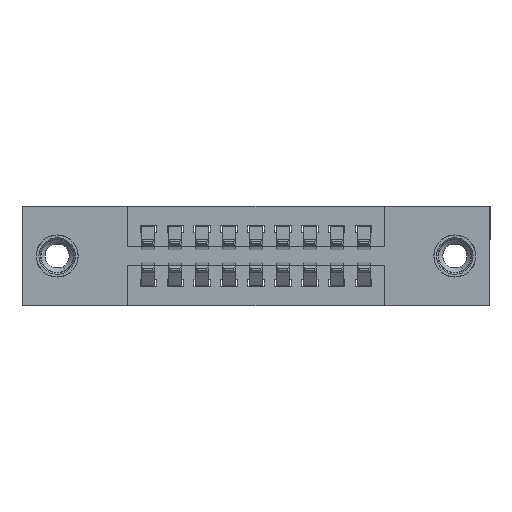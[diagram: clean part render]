
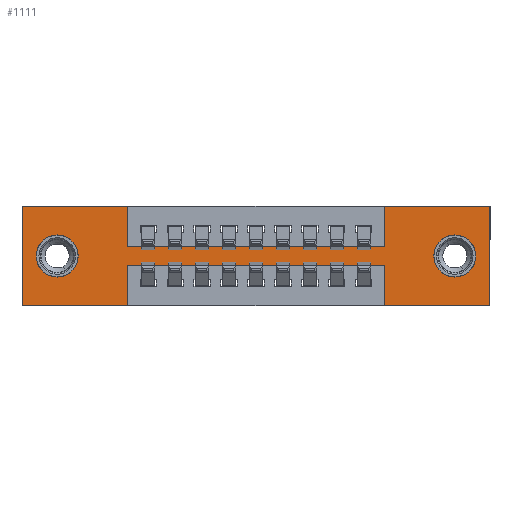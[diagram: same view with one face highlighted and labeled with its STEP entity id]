
A CAD part, front view. The second image highlights one B-rep face of the part: STEP entity #1111.
In plain terms, the highlighted planar face has unit normal (0, -1, 0).
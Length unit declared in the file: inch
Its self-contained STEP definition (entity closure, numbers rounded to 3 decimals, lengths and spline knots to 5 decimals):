
#207 = CARTESIAN_POINT ( 'NONE',  ( 1.3425, 0., -0.37 ) ) ;
#252 = DIRECTION ( 'NONE',  ( 1., 0., 0. ) ) ;
#415 = EDGE_CURVE ( 'NONE', #15424, #10336, #16353, .T. ) ;
#437 = CARTESIAN_POINT ( 'NONE',  ( 1.735, 0., 0. ) ) ;
#595 = ORIENTED_EDGE ( 'NONE', *, *, #5050, .F. ) ;
#692 = CARTESIAN_POINT ( 'NONE',  ( 1.605, 0., -0.263 ) ) ;
#884 = ORIENTED_EDGE ( 'NONE', *, *, #9360, .F. ) ;
#893 = CARTESIAN_POINT ( 'NONE',  ( 1.605, 0., -0.107 ) ) ;
#1111 = ADVANCED_FACE ( 'NONE', ( #7993, #14321, #15718 ), #10980, .T. ) ;
#1293 = AXIS2_PLACEMENT_3D ( 'NONE', #15008, #7419, #13548 ) ;
#1509 = CIRCLE ( 'NONE', #12187, 0.078 ) ;
#1554 = LINE ( 'NONE', #8705, #8069 ) ;
#1849 = CARTESIAN_POINT ( 'NONE',  ( 0., 0., -0.37 ) ) ;
#1929 = CIRCLE ( 'NONE', #10089, 0.078 ) ;
#1953 = VERTEX_POINT ( 'NONE', #10469 ) ;
#1966 = DIRECTION ( 'NONE',  ( -1., 0., 0. ) ) ;
#1985 = DIRECTION ( 'NONE',  ( 0., 0., -1. ) ) ;
#2085 = VECTOR ( 'NONE', #12582, 39.37008 ) ;
#2090 = CARTESIAN_POINT ( 'NONE',  ( 0., 0., -0.37 ) ) ;
#2304 = DIRECTION ( 'NONE',  ( 0., 0., 1. ) ) ;
#2460 = ORIENTED_EDGE ( 'NONE', *, *, #13533, .F. ) ;
#2558 = VECTOR ( 'NONE', #2304, 39.37008 ) ;
#2909 = CARTESIAN_POINT ( 'NONE',  ( 0.3925, 0., -0.22 ) ) ;
#2970 = EDGE_CURVE ( 'NONE', #9337, #15167, #8326, .T. ) ;
#2982 = VERTEX_POINT ( 'NONE', #7199 ) ;
#3263 = DIRECTION ( 'NONE',  ( 0., 0., -1. ) ) ;
#3488 = CARTESIAN_POINT ( 'NONE',  ( 1.605, 0., -0.185 ) ) ;
#3556 = LINE ( 'NONE', #6065, #2558 ) ;
#3629 = DIRECTION ( 'NONE',  ( 0., 0., 1. ) ) ;
#3724 = EDGE_CURVE ( 'NONE', #8773, #15424, #9285, .T. ) ;
#3735 = EDGE_LOOP ( 'NONE', ( #5140, #8130 ) ) ;
#3769 = LINE ( 'NONE', #6509, #15847 ) ;
#3925 = CARTESIAN_POINT ( 'NONE',  ( 1.605, 0., -0.185 ) ) ;
#4067 = EDGE_CURVE ( 'NONE', #6434, #2982, #3769, .T. ) ;
#4069 = DIRECTION ( 'NONE',  ( 0., 1., 0. ) ) ;
#4116 = ORIENTED_EDGE ( 'NONE', *, *, #13829, .F. ) ;
#4537 = VECTOR ( 'NONE', #3263, 39.37008 ) ;
#4695 = LINE ( 'NONE', #15962, #12978 ) ;
#4753 = EDGE_CURVE ( 'NONE', #15594, #6434, #3556, .T. ) ;
#4817 = VECTOR ( 'NONE', #13464, 39.37008 ) ;
#4844 = VECTOR ( 'NONE', #252, 39.37008 ) ;
#4912 = CIRCLE ( 'NONE', #10466, 0.078 ) ;
#5050 = EDGE_CURVE ( 'NONE', #7276, #15594, #13015, .T. ) ;
#5140 = ORIENTED_EDGE ( 'NONE', *, *, #2970, .T. ) ;
#5389 = ORIENTED_EDGE ( 'NONE', *, *, #10647, .F. ) ;
#5525 = CARTESIAN_POINT ( 'NONE',  ( 1.735, 0., -0.37 ) ) ;
#5573 = DIRECTION ( 'NONE',  ( -1., 0., 0. ) ) ;
#5698 = ORIENTED_EDGE ( 'NONE', *, *, #3724, .F. ) ;
#5729 = EDGE_CURVE ( 'NONE', #14629, #13542, #1929, .T. ) ;
#5925 = DIRECTION ( 'NONE',  ( 0., 1., 0. ) ) ;
#6063 = CARTESIAN_POINT ( 'NONE',  ( 0.13, 0., -0.263 ) ) ;
#6065 = CARTESIAN_POINT ( 'NONE',  ( 0., 0., 0. ) ) ;
#6308 = DIRECTION ( 'NONE',  ( 0., 0., -1. ) ) ;
#6364 = ORIENTED_EDGE ( 'NONE', *, *, #415, .F. ) ;
#6434 = VERTEX_POINT ( 'NONE', #12138 ) ;
#6509 = CARTESIAN_POINT ( 'NONE',  ( 0., 0., 0. ) ) ;
#7124 = ORIENTED_EDGE ( 'NONE', *, *, #16138, .F. ) ;
#7172 = CARTESIAN_POINT ( 'NONE',  ( 0.13, 0., -0.185 ) ) ;
#7199 = CARTESIAN_POINT ( 'NONE',  ( 0.3925, 0., 0. ) ) ;
#7224 = CARTESIAN_POINT ( 'NONE',  ( 0.13, 0., -0.107 ) ) ;
#7228 = VECTOR ( 'NONE', #11682, 39.37008 ) ;
#7276 = VERTEX_POINT ( 'NONE', #14597 ) ;
#7419 = DIRECTION ( 'NONE',  ( 0., -1., 0. ) ) ;
#7774 = VERTEX_POINT ( 'NONE', #8724 ) ;
#7982 = ORIENTED_EDGE ( 'NONE', *, *, #4067, .F. ) ;
#7993 = FACE_BOUND ( 'NONE', #3735, .T. ) ;
#8042 = EDGE_LOOP ( 'NONE', ( #13477, #9105 ) ) ;
#8069 = VECTOR ( 'NONE', #3629, 39.37008 ) ;
#8118 = CARTESIAN_POINT ( 'NONE',  ( 0.3925, 0., -0.15 ) ) ;
#8130 = ORIENTED_EDGE ( 'NONE', *, *, #15494, .T. ) ;
#8326 = CIRCLE ( 'NONE', #8721, 0.078 ) ;
#8705 = CARTESIAN_POINT ( 'NONE',  ( 1.3425, 0., 0. ) ) ;
#8721 = AXIS2_PLACEMENT_3D ( 'NONE', #3488, #5925, #1985 ) ;
#8724 = CARTESIAN_POINT ( 'NONE',  ( 1.3425, 0., -0.15 ) ) ;
#8773 = VERTEX_POINT ( 'NONE', #5525 ) ;
#8974 = DIRECTION ( 'NONE',  ( 1., 0., 0. ) ) ;
#9105 = ORIENTED_EDGE ( 'NONE', *, *, #13437, .T. ) ;
#9285 = LINE ( 'NONE', #1849, #12857 ) ;
#9337 = VERTEX_POINT ( 'NONE', #893 ) ;
#9360 = EDGE_CURVE ( 'NONE', #1953, #7774, #16151, .T. ) ;
#9553 = ORIENTED_EDGE ( 'NONE', *, *, #12789, .F. ) ;
#9577 = DIRECTION ( 'NONE',  ( 0., 0., 1. ) ) ;
#9854 = VECTOR ( 'NONE', #1966, 39.37008 ) ;
#9967 = LINE ( 'NONE', #437, #7228 ) ;
#10028 = VECTOR ( 'NONE', #5573, 39.37008 ) ;
#10089 = AXIS2_PLACEMENT_3D ( 'NONE', #15545, #4069, #12922 ) ;
#10190 = CARTESIAN_POINT ( 'NONE',  ( 1.3425, 0., -0.37 ) ) ;
#10324 = ORIENTED_EDGE ( 'NONE', *, *, #4753, .F. ) ;
#10336 = VERTEX_POINT ( 'NONE', #10549 ) ;
#10445 = VERTEX_POINT ( 'NONE', #11400 ) ;
#10466 = AXIS2_PLACEMENT_3D ( 'NONE', #7172, #16143, #9577 ) ;
#10469 = CARTESIAN_POINT ( 'NONE',  ( 0.3925, 0., -0.15 ) ) ;
#10481 = EDGE_LOOP ( 'NONE', ( #9553, #4116, #6364, #5698, #7124, #5389, #2460, #884, #12987, #7982, #10324, #595 ) ) ;
#10549 = CARTESIAN_POINT ( 'NONE',  ( 1.3425, 0., -0.22 ) ) ;
#10647 = EDGE_CURVE ( 'NONE', #10445, #13143, #11479, .T. ) ;
#10894 = DIRECTION ( 'NONE',  ( -1., 0., 0. ) ) ;
#10980 = PLANE ( 'NONE',  #1293 ) ;
#11368 = LINE ( 'NONE', #13121, #10028 ) ;
#11400 = CARTESIAN_POINT ( 'NONE',  ( 1.3425, 0., 0. ) ) ;
#11479 = LINE ( 'NONE', #12153, #4817 ) ;
#11487 = VERTEX_POINT ( 'NONE', #2909 ) ;
#11682 = DIRECTION ( 'NONE',  ( 0., 0., -1. ) ) ;
#11700 = CARTESIAN_POINT ( 'NONE',  ( 0., 0., -0.37 ) ) ;
#12138 = CARTESIAN_POINT ( 'NONE',  ( 0., 0., 0. ) ) ;
#12153 = CARTESIAN_POINT ( 'NONE',  ( 0., 0., 0. ) ) ;
#12187 = AXIS2_PLACEMENT_3D ( 'NONE', #3925, #12509, #6308 ) ;
#12509 = DIRECTION ( 'NONE',  ( 0., 1., 0. ) ) ;
#12582 = DIRECTION ( 'NONE',  ( 0., 0., 1. ) ) ;
#12789 = EDGE_CURVE ( 'NONE', #11487, #7276, #13843, .T. ) ;
#12857 = VECTOR ( 'NONE', #10894, 39.37008 ) ;
#12922 = DIRECTION ( 'NONE',  ( 0., 0., 1. ) ) ;
#12978 = VECTOR ( 'NONE', #15841, 39.37008 ) ;
#12987 = ORIENTED_EDGE ( 'NONE', *, *, #14513, .F. ) ;
#13015 = LINE ( 'NONE', #2090, #9854 ) ;
#13121 = CARTESIAN_POINT ( 'NONE',  ( 0.3925, 0., -0.22 ) ) ;
#13143 = VERTEX_POINT ( 'NONE', #14243 ) ;
#13241 = CARTESIAN_POINT ( 'NONE',  ( 0.3925, 0., -0.37 ) ) ;
#13437 = EDGE_CURVE ( 'NONE', #13542, #14629, #4912, .T. ) ;
#13464 = DIRECTION ( 'NONE',  ( 1., 0., 0. ) ) ;
#13477 = ORIENTED_EDGE ( 'NONE', *, *, #5729, .T. ) ;
#13533 = EDGE_CURVE ( 'NONE', #7774, #10445, #1554, .T. ) ;
#13542 = VERTEX_POINT ( 'NONE', #6063 ) ;
#13548 = DIRECTION ( 'NONE',  ( 0., 0., -1. ) ) ;
#13829 = EDGE_CURVE ( 'NONE', #10336, #11487, #11368, .T. ) ;
#13843 = LINE ( 'NONE', #13241, #4537 ) ;
#14243 = CARTESIAN_POINT ( 'NONE',  ( 1.735, 0., 0. ) ) ;
#14321 = FACE_BOUND ( 'NONE', #8042, .T. ) ;
#14513 = EDGE_CURVE ( 'NONE', #2982, #1953, #4695, .T. ) ;
#14597 = CARTESIAN_POINT ( 'NONE',  ( 0.3925, 0., -0.37 ) ) ;
#14629 = VERTEX_POINT ( 'NONE', #7224 ) ;
#15008 = CARTESIAN_POINT ( 'NONE',  ( 0., 0., -0.37 ) ) ;
#15167 = VERTEX_POINT ( 'NONE', #692 ) ;
#15424 = VERTEX_POINT ( 'NONE', #207 ) ;
#15494 = EDGE_CURVE ( 'NONE', #15167, #9337, #1509, .T. ) ;
#15545 = CARTESIAN_POINT ( 'NONE',  ( 0.13, 0., -0.185 ) ) ;
#15594 = VERTEX_POINT ( 'NONE', #11700 ) ;
#15718 = FACE_OUTER_BOUND ( 'NONE', #10481, .T. ) ;
#15841 = DIRECTION ( 'NONE',  ( 0., 0., -1. ) ) ;
#15847 = VECTOR ( 'NONE', #8974, 39.37008 ) ;
#15962 = CARTESIAN_POINT ( 'NONE',  ( 0.3925, 0., 0. ) ) ;
#16138 = EDGE_CURVE ( 'NONE', #13143, #8773, #9967, .T. ) ;
#16143 = DIRECTION ( 'NONE',  ( 0., 1., 0. ) ) ;
#16151 = LINE ( 'NONE', #8118, #4844 ) ;
#16353 = LINE ( 'NONE', #10190, #2085 ) ;
